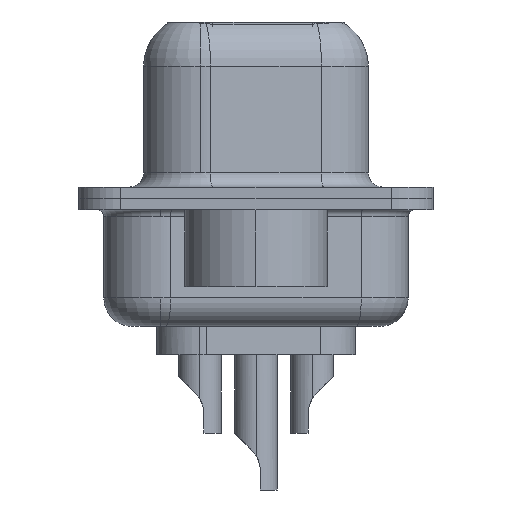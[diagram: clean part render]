
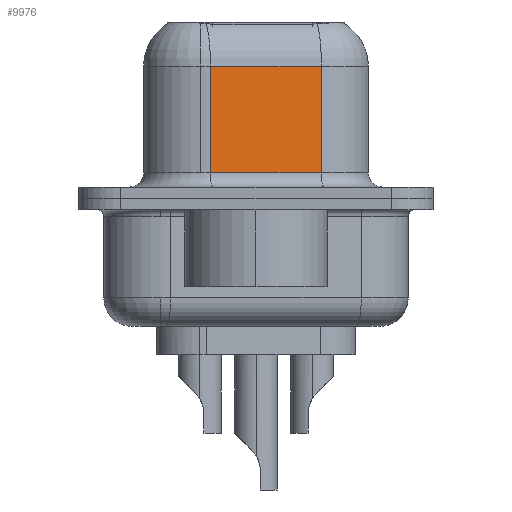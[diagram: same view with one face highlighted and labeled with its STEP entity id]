
A CAD part, left-side view. The second image highlights one B-rep face of the part: STEP entity #9976.
In plain terms, the highlighted planar face has unit normal (-0.985, -0.174, 0).
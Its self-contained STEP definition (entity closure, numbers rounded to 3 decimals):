
#559 = EDGE_LOOP ( 'NONE', ( #18337, #8930, #12042, #11380 ) ) ;
#564 = EDGE_CURVE ( 'NONE', #16841, #18419, #2701, .T. ) ;
#866 = VECTOR ( 'NONE', #18535, 1000. ) ;
#2026 = VERTEX_POINT ( 'NONE', #5977 ) ;
#2701 = LINE ( 'NONE', #11726, #6390 ) ;
#2990 = CARTESIAN_POINT ( 'NONE',  ( 4.38, 1.603, 6.4 ) ) ;
#3903 = CARTESIAN_POINT ( 'NONE',  ( 4.38, 1.603, 4.65 ) ) ;
#5256 = EDGE_CURVE ( 'NONE', #19645, #2026, #9950, .T. ) ;
#5977 = CARTESIAN_POINT ( 'NONE',  ( 4.38, 1.603, 0.9 ) ) ;
#6390 = VECTOR ( 'NONE', #15131, 1000. ) ;
#6453 = CARTESIAN_POINT ( 'NONE',  ( 5.068, -2.297, 0.9 ) ) ;
#6692 = DIRECTION ( 'NONE',  ( 0.174, -0.985, 0. ) ) ;
#7832 = CARTESIAN_POINT ( 'NONE',  ( 5.068, -2.297, 6.4 ) ) ;
#8352 = CARTESIAN_POINT ( 'NONE',  ( 5.068, -2.297, 0.9 ) ) ;
#8724 = VECTOR ( 'NONE', #6692, 1000. ) ;
#8930 = ORIENTED_EDGE ( 'NONE', *, *, #19727, .T. ) ;
#9283 = FACE_OUTER_BOUND ( 'NONE', #559, .T. ) ;
#9760 = PLANE ( 'NONE',  #12103 ) ;
#9950 = LINE ( 'NONE', #2990, #19975 ) ;
#9976 = ADVANCED_FACE ( 'NONE', ( #9283 ), #9760, .F. ) ;
#11380 = ORIENTED_EDGE ( 'NONE', *, *, #13209, .T. ) ;
#11726 = CARTESIAN_POINT ( 'NONE',  ( 5.068, -2.297, 6.4 ) ) ;
#11871 = DIRECTION ( 'NONE',  ( 0., 0., -1. ) ) ;
#12042 = ORIENTED_EDGE ( 'NONE', *, *, #5256, .T. ) ;
#12093 = LINE ( 'NONE', #6453, #8724 ) ;
#12103 = AXIS2_PLACEMENT_3D ( 'NONE', #7832, #14720, #15193 ) ;
#13209 = EDGE_CURVE ( 'NONE', #2026, #18419, #12093, .T. ) ;
#14720 = DIRECTION ( 'NONE',  ( 0.985, 0.174, 0. ) ) ;
#15131 = DIRECTION ( 'NONE',  ( 0., 0., -1. ) ) ;
#15193 = DIRECTION ( 'NONE',  ( -0.174, 0.985, 0. ) ) ;
#16841 = VERTEX_POINT ( 'NONE', #19652 ) ;
#18337 = ORIENTED_EDGE ( 'NONE', *, *, #564, .F. ) ;
#18419 = VERTEX_POINT ( 'NONE', #8352 ) ;
#18535 = DIRECTION ( 'NONE',  ( -0.174, 0.985, 0. ) ) ;
#19645 = VERTEX_POINT ( 'NONE', #3903 ) ;
#19652 = CARTESIAN_POINT ( 'NONE',  ( 5.068, -2.297, 4.65 ) ) ;
#19727 = EDGE_CURVE ( 'NONE', #16841, #19645, #20321, .T. ) ;
#19975 = VECTOR ( 'NONE', #11871, 1000. ) ;
#20321 = LINE ( 'NONE', #23688, #866 ) ;
#23688 = CARTESIAN_POINT ( 'NONE',  ( 5.068, -2.297, 4.65 ) ) ;
